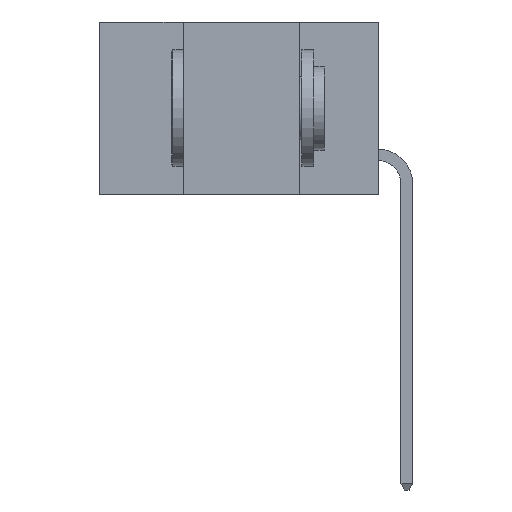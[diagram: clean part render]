
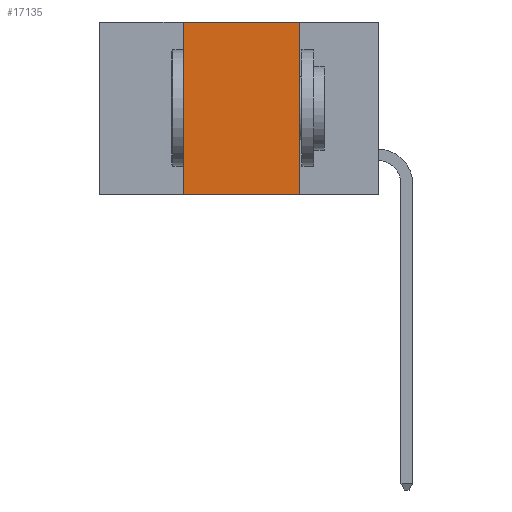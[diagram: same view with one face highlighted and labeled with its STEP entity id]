
A CAD part, left-side view. The second image highlights one B-rep face of the part: STEP entity #17135.
In plain terms, the highlighted planar face has unit normal (-1, 0, 0).
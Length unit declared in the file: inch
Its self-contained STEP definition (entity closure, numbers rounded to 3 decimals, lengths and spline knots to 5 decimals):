
#242 = CARTESIAN_POINT ( 'NONE',  ( 0., 0.42, -0.37 ) ) ;
#2278 = DIRECTION ( 'NONE',  ( 0., 0., 1. ) ) ;
#2621 = VERTEX_POINT ( 'NONE', #7458 ) ;
#2661 = ORIENTED_EDGE ( 'NONE', *, *, #22429, .T. ) ;
#3454 = VECTOR ( 'NONE', #23797, 39.37008 ) ;
#3783 = EDGE_CURVE ( 'NONE', #4823, #11179, #10868, .T. ) ;
#4347 = CARTESIAN_POINT ( 'NONE',  ( 0., 0.6, -0.37 ) ) ;
#4823 = VERTEX_POINT ( 'NONE', #11349 ) ;
#5217 = PLANE ( 'NONE',  #14026 ) ;
#5287 = CARTESIAN_POINT ( 'NONE',  ( 0., 0.17, 0. ) ) ;
#5989 = EDGE_LOOP ( 'NONE', ( #18736, #8429, #22620, #2661 ) ) ;
#6382 = EDGE_CURVE ( 'NONE', #11179, #13815, #14989, .T. ) ;
#7094 = VECTOR ( 'NONE', #19863, 39.37008 ) ;
#7458 = CARTESIAN_POINT ( 'NONE',  ( 0., 0.42, -0.37 ) ) ;
#8429 = ORIENTED_EDGE ( 'NONE', *, *, #3783, .F. ) ;
#9131 = DIRECTION ( 'NONE',  ( 1., 0., 0. ) ) ;
#10455 = LINE ( 'NONE', #4347, #7094 ) ;
#10868 = LINE ( 'NONE', #24091, #14781 ) ;
#11179 = VERTEX_POINT ( 'NONE', #5287 ) ;
#11271 = VECTOR ( 'NONE', #2278, 39.37008 ) ;
#11349 = CARTESIAN_POINT ( 'NONE',  ( 0., 0.42, 0. ) ) ;
#13815 = VERTEX_POINT ( 'NONE', #15865 ) ;
#14026 = AXIS2_PLACEMENT_3D ( 'NONE', #20743, #9131, #22628 ) ;
#14781 = VECTOR ( 'NONE', #24043, 39.37008 ) ;
#14989 = LINE ( 'NONE', #23724, #3454 ) ;
#15865 = CARTESIAN_POINT ( 'NONE',  ( 0., 0.17, -0.37 ) ) ;
#17135 = ADVANCED_FACE ( 'NONE', ( #22565 ), #5217, .F. ) ;
#18736 = ORIENTED_EDGE ( 'NONE', *, *, #6382, .F. ) ;
#19863 = DIRECTION ( 'NONE',  ( 0., -1., 0. ) ) ;
#20743 = CARTESIAN_POINT ( 'NONE',  ( 0., 0.6, 0. ) ) ;
#21531 = LINE ( 'NONE', #242, #11271 ) ;
#22429 = EDGE_CURVE ( 'NONE', #2621, #13815, #10455, .T. ) ;
#22565 = FACE_OUTER_BOUND ( 'NONE', #5989, .T. ) ;
#22620 = ORIENTED_EDGE ( 'NONE', *, *, #24906, .F. ) ;
#22628 = DIRECTION ( 'NONE',  ( 0., 0., -1. ) ) ;
#23724 = CARTESIAN_POINT ( 'NONE',  ( 0., 0.17, -0.37 ) ) ;
#23797 = DIRECTION ( 'NONE',  ( 0., 0., -1. ) ) ;
#24043 = DIRECTION ( 'NONE',  ( 0., -1., 0. ) ) ;
#24091 = CARTESIAN_POINT ( 'NONE',  ( 0., 0.6, 0. ) ) ;
#24906 = EDGE_CURVE ( 'NONE', #2621, #4823, #21531, .T. ) ;
